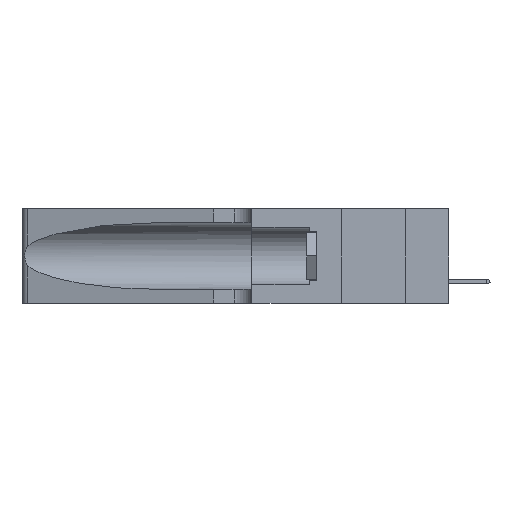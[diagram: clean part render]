
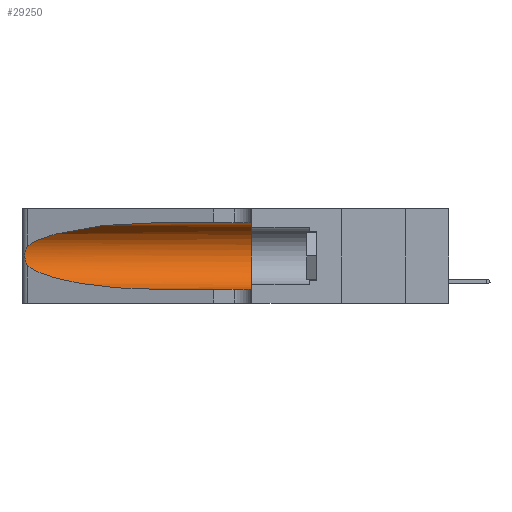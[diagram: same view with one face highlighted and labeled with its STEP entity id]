
A CAD part, left-side view. The second image highlights one B-rep face of the part: STEP entity #29250.
In plain terms, the highlighted cylindrical face has radius 3.308 mm (diameter 6.617 mm), a partial arc.
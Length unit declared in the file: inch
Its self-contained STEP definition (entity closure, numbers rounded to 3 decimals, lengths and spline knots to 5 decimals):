
#1166 = EDGE_CURVE ( 'NONE', #32979, #35864, #32498, .T. ) ;
#2247 = CARTESIAN_POINT ( 'NONE',  ( 0.25856, 1.23593, 0.16098 ) ) ;
#2250 = EDGE_CURVE ( 'NONE', #35864, #4232, #23530, .T. ) ;
#3207 = DIRECTION ( 'NONE',  ( 0., -1., 0. ) ) ;
#3426 = CARTESIAN_POINT ( 'NONE',  ( 0.1305, 0.35, 0.31525 ) ) ;
#3827 = EDGE_CURVE ( 'NONE', #22389, #17896, #26667, .T. ) ;
#3987 = AXIS2_PLACEMENT_3D ( 'NONE', #26902, #31099, #18856 ) ;
#4232 = VERTEX_POINT ( 'NONE', #48151 ) ;
#5597 = CARTESIAN_POINT ( 'NONE',  ( 0.25487, 1.22718, 0.22369 ) ) ;
#5670 = VECTOR ( 'NONE', #3207, 39.37008 ) ;
#5733 = ORIENTED_EDGE ( 'NONE', *, *, #5797, .F. ) ;
#5797 = EDGE_CURVE ( 'NONE', #32979, #46928, #28657, .T. ) ;
#5840 = CARTESIAN_POINT ( 'NONE',  ( 0.1305, 0.72297, 0.05475 ) ) ;
#5891 = EDGE_CURVE ( 'NONE', #46928, #17896, #6310, .T. ) ;
#6310 = CIRCLE ( 'NONE', #39875, 0.13025 ) ;
#7782 = FACE_OUTER_BOUND ( 'NONE', #48490, .T. ) ;
#8184 = ORIENTED_EDGE ( 'NONE', *, *, #3827, .T. ) ;
#8242 = CARTESIAN_POINT ( 'NONE',  ( 0.18966, 0.96281, 0.31525 ) ) ;
#8797 = CYLINDRICAL_SURFACE ( 'NONE', #3987, 0.13025 ) ;
#11134 = CARTESIAN_POINT ( 'NONE',  ( 0.18966, 0.96281, 0.05475 ) ) ;
#11362 = DIRECTION ( 'NONE',  ( 0., 0., 1. ) ) ;
#11657 = CARTESIAN_POINT ( 'NONE',  ( 0.1305, 1.61858, 0.31525 ) ) ;
#11844 = CARTESIAN_POINT ( 'NONE',  ( 0.2373, 1.15595, 0.28018 ) ) ;
#13222 = CARTESIAN_POINT ( 'NONE',  ( 0.25787, 1.23484, 0.2124 ) ) ;
#13775 = CARTESIAN_POINT ( 'NONE',  ( 0.25639, 1.23186, 0.15144 ) ) ;
#14242 = ORIENTED_EDGE ( 'NONE', *, *, #2250, .T. ) ;
#17896 = VERTEX_POINT ( 'NONE', #36134 ) ;
#18407 = CARTESIAN_POINT ( 'NONE',  ( 0.2373, 1.15595, 0.08982 ) ) ;
#18856 = DIRECTION ( 'NONE',  ( 0., 0., -1. ) ) ;
#19823 = CARTESIAN_POINT ( 'NONE',  ( 0.25487, 1.22718, 0.22369 ) ) ;
#20834 = CARTESIAN_POINT ( 'NONE',  ( 0.25639, 1.23184, 0.21858 ) ) ;
#21007 = CARTESIAN_POINT ( 'NONE',  ( 0.25487, 1.22718, 0.14631 ) ) ;
#22389 = VERTEX_POINT ( 'NONE', #5840 ) ;
#22777 = CARTESIAN_POINT ( 'NONE',  ( 0.1305, 0.72297, 0.05475 ) ) ;
#23530 = B_SPLINE_CURVE_WITH_KNOTS ( 'NONE', 3,
 ( #5597, #48008, #20834, #13222, #47826, #24672, #44120, #40591, #25189, #2247, #33013, #13775, #40780, #21007 ),
 .UNSPECIFIED., .F., .F.,
 ( 4, 2, 2, 2, 2, 2, 4 ),
 ( 0., 0.00027, 0.00053, 0.00107, 0.0016, 0.00187, 0.00214 ),
 .UNSPECIFIED. ) ;
#23742 = CARTESIAN_POINT ( 'NONE',  ( 0.1305, 1.61858, 0.05475 ) ) ;
#24672 = CARTESIAN_POINT ( 'NONE',  ( 0.26018, 1.23835, 0.19895 ) ) ;
#25189 = CARTESIAN_POINT ( 'NONE',  ( 0.26017, 1.23833, 0.17102 ) ) ;
#26667 = LINE ( 'NONE', #23742, #46584 ) ;
#26902 = CARTESIAN_POINT ( 'NONE',  ( 0.1305, 1.61858, 0.185 ) ) ;
#28657 = LINE ( 'NONE', #11657, #5670 ) ;
#28741 = ORIENTED_EDGE ( 'NONE', *, *, #1166, .T. ) ;
#29250 = ADVANCED_FACE ( 'NONE', ( #7782 ), #8797, .F. ) ;
#29466 = ORIENTED_EDGE ( 'NONE', *, *, #5891, .F. ) ;
#31099 = DIRECTION ( 'NONE',  ( 0., -1., 0. ) ) ;
#31905 = EDGE_CURVE ( 'NONE', #4232, #22389, #46743, .T. ) ;
#32498 =( BOUNDED_CURVE ( )  B_SPLINE_CURVE ( 3, ( #46748, #8242, #11844, #38836 ),
 .UNSPECIFIED., .F., .F. ) 
 B_SPLINE_CURVE_WITH_KNOTS ( ( 4, 4 ),
 ( 1.5708, 2.84003 ),
 .UNSPECIFIED. ) 
 CURVE ( )  GEOMETRIC_REPRESENTATION_ITEM ( )  RATIONAL_B_SPLINE_CURVE ( ( 1., 0.87, 0.87, 1. ) ) 
 REPRESENTATION_ITEM ( '' )  );
#32979 = VERTEX_POINT ( 'NONE', #33809 ) ;
#33013 = CARTESIAN_POINT ( 'NONE',  ( 0.25789, 1.23486, 0.15765 ) ) ;
#33809 = CARTESIAN_POINT ( 'NONE',  ( 0.1305, 0.72297, 0.31525 ) ) ;
#35091 = DIRECTION ( 'NONE',  ( 0., -1., 0. ) ) ;
#35528 = CARTESIAN_POINT ( 'NONE',  ( 0.1305, 0.35, 0.185 ) ) ;
#35864 = VERTEX_POINT ( 'NONE', #19823 ) ;
#36134 = CARTESIAN_POINT ( 'NONE',  ( 0.1305, 0.35, 0.05475 ) ) ;
#37613 = CARTESIAN_POINT ( 'NONE',  ( 0.25487, 1.22718, 0.14631 ) ) ;
#38836 = CARTESIAN_POINT ( 'NONE',  ( 0.25487, 1.22718, 0.22369 ) ) ;
#39875 = AXIS2_PLACEMENT_3D ( 'NONE', #35528, #42970, #11362 ) ;
#40591 = CARTESIAN_POINT ( 'NONE',  ( 0.26075, 1.23896, 0.178 ) ) ;
#40780 = CARTESIAN_POINT ( 'NONE',  ( 0.25555, 1.22993, 0.14849 ) ) ;
#42497 = ORIENTED_EDGE ( 'NONE', *, *, #31905, .T. ) ;
#42970 = DIRECTION ( 'NONE',  ( 0., 1., 0. ) ) ;
#44120 = CARTESIAN_POINT ( 'NONE',  ( 0.26075, 1.23896, 0.19203 ) ) ;
#46584 = VECTOR ( 'NONE', #35091, 39.37008 ) ;
#46743 =( BOUNDED_CURVE ( )  B_SPLINE_CURVE ( 3, ( #37613, #18407, #11134, #22777 ),
 .UNSPECIFIED., .F., .F. ) 
 B_SPLINE_CURVE_WITH_KNOTS ( ( 4, 4 ),
 ( 3.44316, 4.71239 ),
 .UNSPECIFIED. ) 
 CURVE ( )  GEOMETRIC_REPRESENTATION_ITEM ( )  RATIONAL_B_SPLINE_CURVE ( ( 1., 0.87, 0.87, 1. ) ) 
 REPRESENTATION_ITEM ( '' )  );
#46748 = CARTESIAN_POINT ( 'NONE',  ( 0.1305, 0.72297, 0.31525 ) ) ;
#46928 = VERTEX_POINT ( 'NONE', #3426 ) ;
#47826 = CARTESIAN_POINT ( 'NONE',  ( 0.25854, 1.2359, 0.20912 ) ) ;
#48008 = CARTESIAN_POINT ( 'NONE',  ( 0.25555, 1.22994, 0.2215 ) ) ;
#48151 = CARTESIAN_POINT ( 'NONE',  ( 0.25487, 1.22718, 0.14631 ) ) ;
#48490 = EDGE_LOOP ( 'NONE', ( #28741, #14242, #42497, #8184, #29466, #5733 ) ) ;
